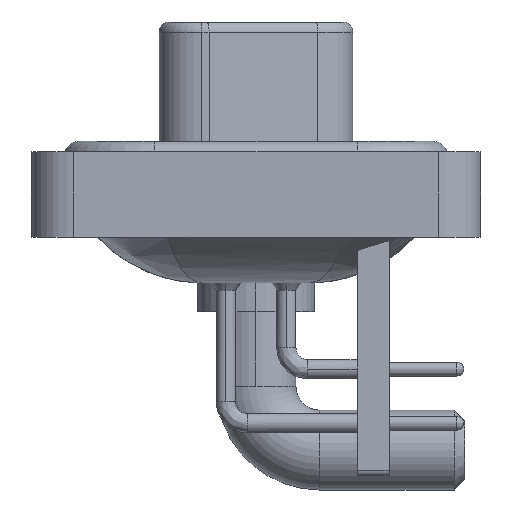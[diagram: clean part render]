
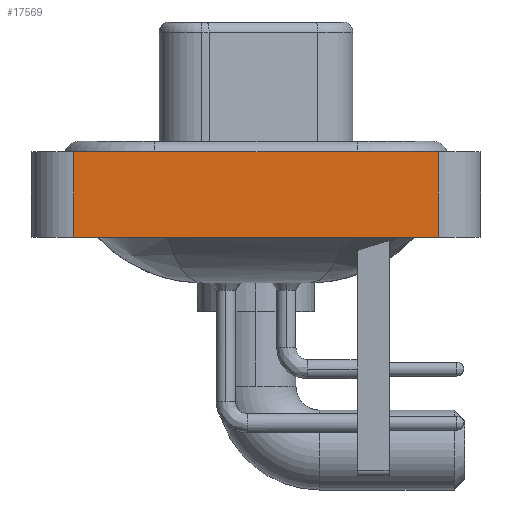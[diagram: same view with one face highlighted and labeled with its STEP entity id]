
A CAD part, left-side view. The second image highlights one B-rep face of the part: STEP entity #17569.
In plain terms, the highlighted planar face has unit normal (-1, 0, 0).
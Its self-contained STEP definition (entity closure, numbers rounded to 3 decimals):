
#123 = ORIENTED_EDGE ( 'NONE', *, *, #4115, .F. ) ;
#394 = EDGE_CURVE ( 'NONE', #24067, #16554, #3076, .T. ) ;
#478 = DIRECTION ( 'NONE',  ( 0., 0., 1. ) ) ;
#1325 = DIRECTION ( 'NONE',  ( 0., -1., 0. ) ) ;
#1747 = CARTESIAN_POINT ( 'NONE',  ( -7.3, 8.55, 0.4 ) ) ;
#1946 = CARTESIAN_POINT ( 'NONE',  ( -7.3, -8.55, -3.6 ) ) ;
#3076 = LINE ( 'NONE', #9474, #19216 ) ;
#3165 = DIRECTION ( 'NONE',  ( -1., 0., 0. ) ) ;
#3705 = DIRECTION ( 'NONE',  ( 0., 0., 1. ) ) ;
#4115 = EDGE_CURVE ( 'NONE', #26638, #24067, #16994, .T. ) ;
#5350 = PLANE ( 'NONE',  #26190 ) ;
#5621 = VECTOR ( 'NONE', #478, 1000. ) ;
#6247 = EDGE_CURVE ( 'NONE', #26638, #23775, #16790, .T. ) ;
#7518 = EDGE_LOOP ( 'NONE', ( #24878, #20415, #123, #20484 ) ) ;
#7758 = FACE_OUTER_BOUND ( 'NONE', #7518, .T. ) ;
#9474 = CARTESIAN_POINT ( 'NONE',  ( -7.3, -8.55, 0.4 ) ) ;
#10976 = CARTESIAN_POINT ( 'NONE',  ( -7.3, -8.55, -3.6 ) ) ;
#11209 = CARTESIAN_POINT ( 'NONE',  ( -7.3, 8.55, -3.6 ) ) ;
#13015 = DIRECTION ( 'NONE',  ( 0., -1., 0. ) ) ;
#15690 = CARTESIAN_POINT ( 'NONE',  ( -7.3, -8.55, -3.6 ) ) ;
#16367 = VECTOR ( 'NONE', #3705, 1000. ) ;
#16554 = VERTEX_POINT ( 'NONE', #25973 ) ;
#16790 = LINE ( 'NONE', #10976, #24256 ) ;
#16994 = LINE ( 'NONE', #19282, #5621 ) ;
#17569 = ADVANCED_FACE ( 'NONE', ( #7758 ), #5350, .T. ) ;
#19216 = VECTOR ( 'NONE', #1325, 1000. ) ;
#19282 = CARTESIAN_POINT ( 'NONE',  ( -7.3, 8.55, -3.6 ) ) ;
#20415 = ORIENTED_EDGE ( 'NONE', *, *, #394, .F. ) ;
#20484 = ORIENTED_EDGE ( 'NONE', *, *, #6247, .T. ) ;
#23775 = VERTEX_POINT ( 'NONE', #15690 ) ;
#23870 = CARTESIAN_POINT ( 'NONE',  ( -7.3, -8.55, -3.6 ) ) ;
#24067 = VERTEX_POINT ( 'NONE', #1747 ) ;
#24133 = DIRECTION ( 'NONE',  ( 0., 0., 1. ) ) ;
#24256 = VECTOR ( 'NONE', #13015, 1000. ) ;
#24670 = LINE ( 'NONE', #1946, #16367 ) ;
#24878 = ORIENTED_EDGE ( 'NONE', *, *, #24950, .T. ) ;
#24950 = EDGE_CURVE ( 'NONE', #23775, #16554, #24670, .T. ) ;
#25973 = CARTESIAN_POINT ( 'NONE',  ( -7.3, -8.55, 0.4 ) ) ;
#26190 = AXIS2_PLACEMENT_3D ( 'NONE', #23870, #3165, #24133 ) ;
#26638 = VERTEX_POINT ( 'NONE', #11209 ) ;
